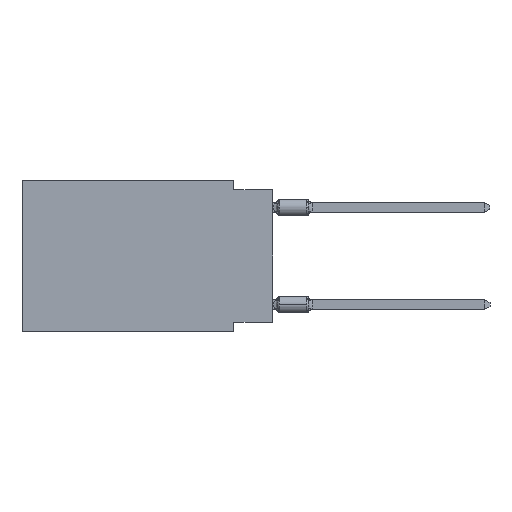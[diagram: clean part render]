
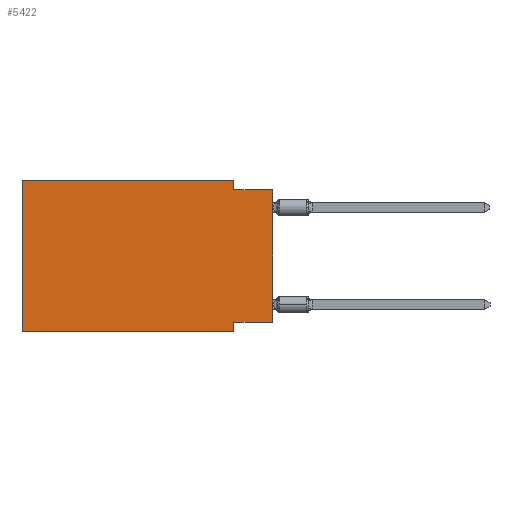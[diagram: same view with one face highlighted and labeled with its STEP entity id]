
A CAD part, left-side view. The second image highlights one B-rep face of the part: STEP entity #5422.
In plain terms, the highlighted planar face has unit normal (-1, 0, 0).
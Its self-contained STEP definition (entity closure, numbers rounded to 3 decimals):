
#521 = LINE ( 'NONE', #23384, #2197 ) ;
#1225 = DIRECTION ( 'NONE',  ( 0., -1., 0. ) ) ;
#1462 = VERTEX_POINT ( 'NONE', #17135 ) ;
#1588 = PLANE ( 'NONE',  #6011 ) ;
#1781 = ORIENTED_EDGE ( 'NONE', *, *, #4223, .F. ) ;
#2197 = VECTOR ( 'NONE', #9675, 1000. ) ;
#2515 = EDGE_LOOP ( 'NONE', ( #13199, #8833, #3751, #3283, #23159, #5525, #1781, #2908 ) ) ;
#2583 = VERTEX_POINT ( 'NONE', #5037 ) ;
#2624 = VERTEX_POINT ( 'NONE', #28246 ) ;
#2667 = VECTOR ( 'NONE', #25325, 1000. ) ;
#2908 = ORIENTED_EDGE ( 'NONE', *, *, #25369, .F. ) ;
#3283 = ORIENTED_EDGE ( 'NONE', *, *, #5710, .F. ) ;
#3442 = EDGE_CURVE ( 'NONE', #2583, #17684, #4960, .T. ) ;
#3708 = CARTESIAN_POINT ( 'NONE',  ( 0., 16.383, -9.906 ) ) ;
#3751 = ORIENTED_EDGE ( 'NONE', *, *, #3442, .F. ) ;
#3831 = FACE_OUTER_BOUND ( 'NONE', #2515, .T. ) ;
#4027 = VERTEX_POINT ( 'NONE', #7466 ) ;
#4223 = EDGE_CURVE ( 'NONE', #24654, #2624, #27662, .T. ) ;
#4960 = LINE ( 'NONE', #20057, #23439 ) ;
#5037 = CARTESIAN_POINT ( 'NONE',  ( 0., 2.54, 0. ) ) ;
#5422 = ADVANCED_FACE ( 'NONE', ( #3831 ), #1588, .F. ) ;
#5525 = ORIENTED_EDGE ( 'NONE', *, *, #20467, .T. ) ;
#5677 = VECTOR ( 'NONE', #18268, 1000. ) ;
#5710 = EDGE_CURVE ( 'NONE', #29530, #2583, #521, .T. ) ;
#6011 = AXIS2_PLACEMENT_3D ( 'NONE', #10890, #21915, #8193 ) ;
#6032 = EDGE_CURVE ( 'NONE', #20166, #4027, #9340, .T. ) ;
#7466 = CARTESIAN_POINT ( 'NONE',  ( 0., 0., -0.635 ) ) ;
#8193 = DIRECTION ( 'NONE',  ( 0., 0., -1. ) ) ;
#8666 = LINE ( 'NONE', #3708, #26335 ) ;
#8833 = ORIENTED_EDGE ( 'NONE', *, *, #18303, .F. ) ;
#9326 = CARTESIAN_POINT ( 'NONE',  ( 0., 16.383, 0. ) ) ;
#9340 = LINE ( 'NONE', #9793, #28247 ) ;
#9492 = DIRECTION ( 'NONE',  ( 0., 0., 1. ) ) ;
#9675 = DIRECTION ( 'NONE',  ( 0., -1., 0. ) ) ;
#9793 = CARTESIAN_POINT ( 'NONE',  ( 0., 0., 0. ) ) ;
#10890 = CARTESIAN_POINT ( 'NONE',  ( 0., 16.383, 0. ) ) ;
#11731 = LINE ( 'NONE', #9326, #16708 ) ;
#12396 = VECTOR ( 'NONE', #1225, 1000. ) ;
#12505 = LINE ( 'NONE', #19273, #12396 ) ;
#13031 = DIRECTION ( 'NONE',  ( 0., -1., 0. ) ) ;
#13123 = DIRECTION ( 'NONE',  ( 0., 0., -1. ) ) ;
#13199 = ORIENTED_EDGE ( 'NONE', *, *, #6032, .T. ) ;
#16106 = LINE ( 'NONE', #25777, #2667 ) ;
#16708 = VECTOR ( 'NONE', #18489, 1000. ) ;
#17135 = CARTESIAN_POINT ( 'NONE',  ( 0., 16.383, -9.906 ) ) ;
#17684 = VERTEX_POINT ( 'NONE', #21145 ) ;
#18268 = DIRECTION ( 'NONE',  ( 0., 0., -1. ) ) ;
#18303 = EDGE_CURVE ( 'NONE', #17684, #4027, #12505, .T. ) ;
#18310 = CARTESIAN_POINT ( 'NONE',  ( 0., 0., -9.271 ) ) ;
#18489 = DIRECTION ( 'NONE',  ( 0., 0., 1. ) ) ;
#18578 = EDGE_CURVE ( 'NONE', #1462, #29530, #11731, .T. ) ;
#19273 = CARTESIAN_POINT ( 'NONE',  ( 0., 0., -0.635 ) ) ;
#20057 = CARTESIAN_POINT ( 'NONE',  ( 0., 2.54, 0. ) ) ;
#20166 = VERTEX_POINT ( 'NONE', #18310 ) ;
#20399 = CARTESIAN_POINT ( 'NONE',  ( 0., 2.54, -9.906 ) ) ;
#20467 = EDGE_CURVE ( 'NONE', #1462, #2624, #8666, .T. ) ;
#21145 = CARTESIAN_POINT ( 'NONE',  ( 0., 2.54, -0.635 ) ) ;
#21915 = DIRECTION ( 'NONE',  ( 1., 0., 0. ) ) ;
#23159 = ORIENTED_EDGE ( 'NONE', *, *, #18578, .F. ) ;
#23384 = CARTESIAN_POINT ( 'NONE',  ( 0., 16.383, 0. ) ) ;
#23439 = VECTOR ( 'NONE', #13123, 1000. ) ;
#24454 = CARTESIAN_POINT ( 'NONE',  ( 0., 16.383, 0. ) ) ;
#24654 = VERTEX_POINT ( 'NONE', #28151 ) ;
#25325 = DIRECTION ( 'NONE',  ( 0., 1., 0. ) ) ;
#25369 = EDGE_CURVE ( 'NONE', #20166, #24654, #16106, .T. ) ;
#25777 = CARTESIAN_POINT ( 'NONE',  ( 0., 0., -9.271 ) ) ;
#26335 = VECTOR ( 'NONE', #13031, 1000. ) ;
#27662 = LINE ( 'NONE', #20399, #5677 ) ;
#28151 = CARTESIAN_POINT ( 'NONE',  ( 0., 2.54, -9.271 ) ) ;
#28246 = CARTESIAN_POINT ( 'NONE',  ( 0., 2.54, -9.906 ) ) ;
#28247 = VECTOR ( 'NONE', #9492, 1000. ) ;
#29530 = VERTEX_POINT ( 'NONE', #24454 ) ;
